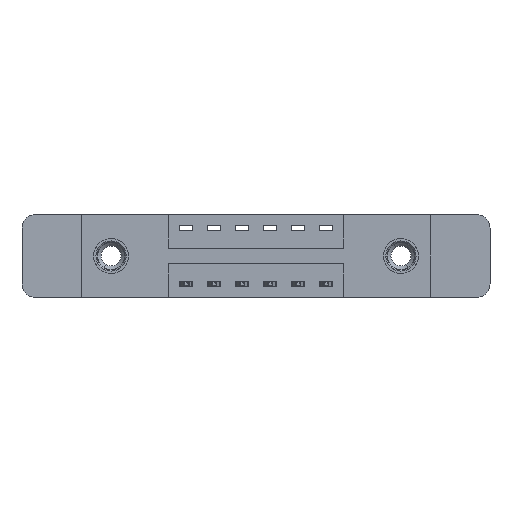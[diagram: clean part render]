
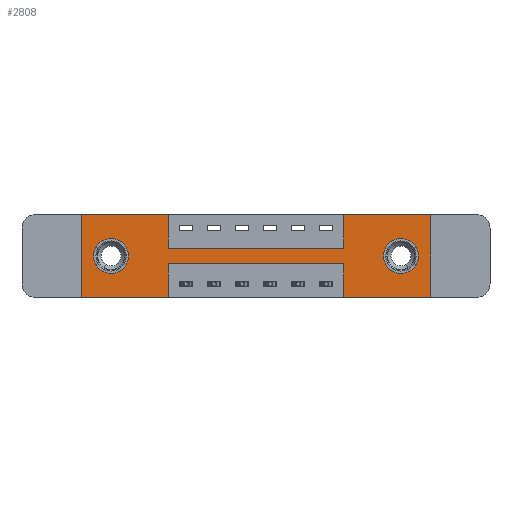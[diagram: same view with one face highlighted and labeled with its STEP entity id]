
A CAD part, front view. The second image highlights one B-rep face of the part: STEP entity #2808.
In plain terms, the highlighted planar face has unit normal (0, -1, 0).
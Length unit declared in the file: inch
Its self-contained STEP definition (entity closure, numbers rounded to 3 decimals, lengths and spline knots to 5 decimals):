
#11 = LINE ( 'NONE', #8748, #278 ) ;
#76 = CIRCLE ( 'NONE', #1911, 0.078 ) ;
#87 = EDGE_CURVE ( 'NONE', #12521, #4204, #11429, .T. ) ;
#151 = DIRECTION ( 'NONE',  ( 0., 1., 0. ) ) ;
#193 = CARTESIAN_POINT ( 'NONE',  ( 0.1325, 0., -0.263 ) ) ;
#278 = VECTOR ( 'NONE', #4473, 39.37008 ) ;
#501 = DIRECTION ( 'NONE',  ( 0., 0., 1. ) ) ;
#564 = ORIENTED_EDGE ( 'NONE', *, *, #10499, .F. ) ;
#595 = DIRECTION ( 'NONE',  ( 0., 0., -1. ) ) ;
#602 = CARTESIAN_POINT ( 'NONE',  ( 0., 0., 0. ) ) ;
#633 = DIRECTION ( 'NONE',  ( 0., 0., -1. ) ) ;
#649 = EDGE_CURVE ( 'NONE', #11373, #13900, #1404, .T. ) ;
#768 = ORIENTED_EDGE ( 'NONE', *, *, #13233, .F. ) ;
#831 = EDGE_CURVE ( 'NONE', #4204, #5177, #8608, .T. ) ;
#1031 = DIRECTION ( 'NONE',  ( 0., 1., 0. ) ) ;
#1092 = CARTESIAN_POINT ( 'NONE',  ( 0.3875, 0., -0.37 ) ) ;
#1094 = ORIENTED_EDGE ( 'NONE', *, *, #87, .F. ) ;
#1285 = ORIENTED_EDGE ( 'NONE', *, *, #5003, .F. ) ;
#1404 = LINE ( 'NONE', #7046, #5067 ) ;
#1556 = CARTESIAN_POINT ( 'NONE',  ( 0.1325, 0., -0.107 ) ) ;
#1605 = CARTESIAN_POINT ( 'NONE',  ( 0.3875, 0., -0.37 ) ) ;
#1806 = CARTESIAN_POINT ( 'NONE',  ( 1.56, 0., 0. ) ) ;
#1860 = DIRECTION ( 'NONE',  ( 0., 0., 1. ) ) ;
#1911 = AXIS2_PLACEMENT_3D ( 'NONE', #4005, #9573, #633 ) ;
#1991 = VECTOR ( 'NONE', #10733, 39.37008 ) ;
#2243 = VECTOR ( 'NONE', #10345, 39.37008 ) ;
#2253 = CARTESIAN_POINT ( 'NONE',  ( 0.1325, 0., -0.185 ) ) ;
#2271 = CIRCLE ( 'NONE', #4801, 0.078 ) ;
#2304 = CARTESIAN_POINT ( 'NONE',  ( 1.1725, 0., -0.37 ) ) ;
#2391 = CARTESIAN_POINT ( 'NONE',  ( 0., 0., 0. ) ) ;
#2398 = VECTOR ( 'NONE', #1860, 39.37008 ) ;
#2683 = EDGE_CURVE ( 'NONE', #5656, #12521, #10015, .T. ) ;
#2749 = DIRECTION ( 'NONE',  ( 0., 0., 1. ) ) ;
#2750 = EDGE_CURVE ( 'NONE', #9265, #10289, #2271, .T. ) ;
#2808 = ADVANCED_FACE ( 'NONE', ( #12226, #4629, #8826 ), #5706, .T. ) ;
#2895 = CARTESIAN_POINT ( 'NONE',  ( 1.1725, 0., -0.37 ) ) ;
#2900 = LINE ( 'NONE', #8113, #8766 ) ;
#3069 = ORIENTED_EDGE ( 'NONE', *, *, #11145, .F. ) ;
#3147 = LINE ( 'NONE', #11815, #1991 ) ;
#3184 = DIRECTION ( 'NONE',  ( 1., 0., 0. ) ) ;
#3343 = VERTEX_POINT ( 'NONE', #1806 ) ;
#3462 = EDGE_CURVE ( 'NONE', #5138, #10152, #9822, .T. ) ;
#3549 = CARTESIAN_POINT ( 'NONE',  ( 0., 0., -0.37 ) ) ;
#3820 = CARTESIAN_POINT ( 'NONE',  ( 0.1325, 0., -0.185 ) ) ;
#3971 = CIRCLE ( 'NONE', #13819, 0.078 ) ;
#4005 = CARTESIAN_POINT ( 'NONE',  ( 1.4275, 0., -0.185 ) ) ;
#4066 = CARTESIAN_POINT ( 'NONE',  ( 1.1725, 0., -0.15 ) ) ;
#4204 = VERTEX_POINT ( 'NONE', #2391 ) ;
#4255 = CARTESIAN_POINT ( 'NONE',  ( 1.4275, 0., -0.185 ) ) ;
#4313 = ORIENTED_EDGE ( 'NONE', *, *, #9751, .T. ) ;
#4335 = AXIS2_PLACEMENT_3D ( 'NONE', #3820, #8167, #2749 ) ;
#4473 = DIRECTION ( 'NONE',  ( -1., 0., 0. ) ) ;
#4498 = CARTESIAN_POINT ( 'NONE',  ( 1.1725, 0., -0.22 ) ) ;
#4629 = FACE_BOUND ( 'NONE', #13347, .T. ) ;
#4801 = AXIS2_PLACEMENT_3D ( 'NONE', #4255, #1031, #9770 ) ;
#4922 = CARTESIAN_POINT ( 'NONE',  ( 0.3875, 0., -0.15 ) ) ;
#5003 = EDGE_CURVE ( 'NONE', #9957, #11083, #3147, .T. ) ;
#5067 = VECTOR ( 'NONE', #9248, 39.37008 ) ;
#5121 = DIRECTION ( 'NONE',  ( 0., 0., 1. ) ) ;
#5138 = VERTEX_POINT ( 'NONE', #1556 ) ;
#5177 = VERTEX_POINT ( 'NONE', #10013 ) ;
#5276 = VECTOR ( 'NONE', #5121, 39.37008 ) ;
#5452 = EDGE_CURVE ( 'NONE', #5177, #11373, #13965, .T. ) ;
#5534 = ORIENTED_EDGE ( 'NONE', *, *, #3462, .T. ) ;
#5640 = EDGE_CURVE ( 'NONE', #9316, #3343, #9184, .T. ) ;
#5656 = VERTEX_POINT ( 'NONE', #1605 ) ;
#5706 = PLANE ( 'NONE',  #12796 ) ;
#6172 = CARTESIAN_POINT ( 'NONE',  ( 1.1725, 0., 0. ) ) ;
#6200 = CARTESIAN_POINT ( 'NONE',  ( 0., 0., 0. ) ) ;
#7046 = CARTESIAN_POINT ( 'NONE',  ( 0.3875, 0., -0.15 ) ) ;
#7402 = CARTESIAN_POINT ( 'NONE',  ( 0.3875, 0., 0. ) ) ;
#7633 = ORIENTED_EDGE ( 'NONE', *, *, #9558, .F. ) ;
#7893 = DIRECTION ( 'NONE',  ( 0., -1., 0. ) ) ;
#8072 = CARTESIAN_POINT ( 'NONE',  ( 0., 0., -0.37 ) ) ;
#8106 = ORIENTED_EDGE ( 'NONE', *, *, #5640, .F. ) ;
#8113 = CARTESIAN_POINT ( 'NONE',  ( 1.56, 0., 0. ) ) ;
#8131 = EDGE_CURVE ( 'NONE', #14210, #9128, #11, .T. ) ;
#8167 = DIRECTION ( 'NONE',  ( 0., 1., 0. ) ) ;
#8466 = EDGE_LOOP ( 'NONE', ( #11600, #10038 ) ) ;
#8530 = DIRECTION ( 'NONE',  ( 0., 0., 1. ) ) ;
#8608 = LINE ( 'NONE', #12999, #13544 ) ;
#8670 = ORIENTED_EDGE ( 'NONE', *, *, #8131, .F. ) ;
#8748 = CARTESIAN_POINT ( 'NONE',  ( 0.3875, 0., -0.22 ) ) ;
#8766 = VECTOR ( 'NONE', #595, 39.37008 ) ;
#8826 = FACE_OUTER_BOUND ( 'NONE', #11075, .T. ) ;
#9128 = VERTEX_POINT ( 'NONE', #11516 ) ;
#9184 = LINE ( 'NONE', #602, #2243 ) ;
#9248 = DIRECTION ( 'NONE',  ( 1., 0., 0. ) ) ;
#9261 = CARTESIAN_POINT ( 'NONE',  ( 1.4275, 0., -0.107 ) ) ;
#9265 = VERTEX_POINT ( 'NONE', #10780 ) ;
#9288 = LINE ( 'NONE', #6172, #2398 ) ;
#9316 = VERTEX_POINT ( 'NONE', #10856 ) ;
#9350 = ORIENTED_EDGE ( 'NONE', *, *, #649, .F. ) ;
#9524 = VECTOR ( 'NONE', #11796, 39.37008 ) ;
#9558 = EDGE_CURVE ( 'NONE', #3343, #9957, #2900, .T. ) ;
#9573 = DIRECTION ( 'NONE',  ( 0., 1., 0. ) ) ;
#9619 = ORIENTED_EDGE ( 'NONE', *, *, #831, .F. ) ;
#9751 = EDGE_CURVE ( 'NONE', #10152, #5138, #3971, .T. ) ;
#9770 = DIRECTION ( 'NONE',  ( 0., 0., -1. ) ) ;
#9773 = VECTOR ( 'NONE', #8530, 39.37008 ) ;
#9822 = CIRCLE ( 'NONE', #4335, 0.078 ) ;
#9845 = EDGE_CURVE ( 'NONE', #10289, #9265, #76, .T. ) ;
#9957 = VERTEX_POINT ( 'NONE', #13978 ) ;
#10013 = CARTESIAN_POINT ( 'NONE',  ( 0.3875, 0., 0. ) ) ;
#10015 = LINE ( 'NONE', #8072, #11485 ) ;
#10038 = ORIENTED_EDGE ( 'NONE', *, *, #2750, .T. ) ;
#10152 = VERTEX_POINT ( 'NONE', #193 ) ;
#10227 = ORIENTED_EDGE ( 'NONE', *, *, #2683, .F. ) ;
#10289 = VERTEX_POINT ( 'NONE', #9261 ) ;
#10345 = DIRECTION ( 'NONE',  ( 1., 0., 0. ) ) ;
#10499 = EDGE_CURVE ( 'NONE', #11083, #14210, #11843, .T. ) ;
#10733 = DIRECTION ( 'NONE',  ( -1., 0., 0. ) ) ;
#10780 = CARTESIAN_POINT ( 'NONE',  ( 1.4275, 0., -0.263 ) ) ;
#10856 = CARTESIAN_POINT ( 'NONE',  ( 1.1725, 0., 0. ) ) ;
#10978 = DIRECTION ( 'NONE',  ( 0., 0., -1. ) ) ;
#11075 = EDGE_LOOP ( 'NONE', ( #768, #8670, #564, #1285, #7633, #8106, #3069, #9350, #13689, #9619, #1094, #10227 ) ) ;
#11083 = VERTEX_POINT ( 'NONE', #2304 ) ;
#11145 = EDGE_CURVE ( 'NONE', #13900, #9316, #9288, .T. ) ;
#11169 = CARTESIAN_POINT ( 'NONE',  ( 0., 0., -0.37 ) ) ;
#11204 = DIRECTION ( 'NONE',  ( 0., 0., -1. ) ) ;
#11240 = DIRECTION ( 'NONE',  ( -1., 0., 0. ) ) ;
#11373 = VERTEX_POINT ( 'NONE', #4922 ) ;
#11429 = LINE ( 'NONE', #6200, #5276 ) ;
#11485 = VECTOR ( 'NONE', #11240, 39.37008 ) ;
#11516 = CARTESIAN_POINT ( 'NONE',  ( 0.3875, 0., -0.22 ) ) ;
#11600 = ORIENTED_EDGE ( 'NONE', *, *, #9845, .T. ) ;
#11796 = DIRECTION ( 'NONE',  ( 0., 0., -1. ) ) ;
#11815 = CARTESIAN_POINT ( 'NONE',  ( 0., 0., -0.37 ) ) ;
#11843 = LINE ( 'NONE', #2895, #9773 ) ;
#12226 = FACE_BOUND ( 'NONE', #8466, .T. ) ;
#12521 = VERTEX_POINT ( 'NONE', #11169 ) ;
#12796 = AXIS2_PLACEMENT_3D ( 'NONE', #3549, #7893, #11204 ) ;
#12999 = CARTESIAN_POINT ( 'NONE',  ( 0., 0., 0. ) ) ;
#13220 = VECTOR ( 'NONE', #10978, 39.37008 ) ;
#13233 = EDGE_CURVE ( 'NONE', #9128, #5656, #14161, .T. ) ;
#13347 = EDGE_LOOP ( 'NONE', ( #5534, #4313 ) ) ;
#13544 = VECTOR ( 'NONE', #3184, 39.37008 ) ;
#13689 = ORIENTED_EDGE ( 'NONE', *, *, #5452, .F. ) ;
#13819 = AXIS2_PLACEMENT_3D ( 'NONE', #2253, #151, #501 ) ;
#13900 = VERTEX_POINT ( 'NONE', #4066 ) ;
#13965 = LINE ( 'NONE', #7402, #9524 ) ;
#13978 = CARTESIAN_POINT ( 'NONE',  ( 1.56, 0., -0.37 ) ) ;
#14161 = LINE ( 'NONE', #1092, #13220 ) ;
#14210 = VERTEX_POINT ( 'NONE', #4498 ) ;
